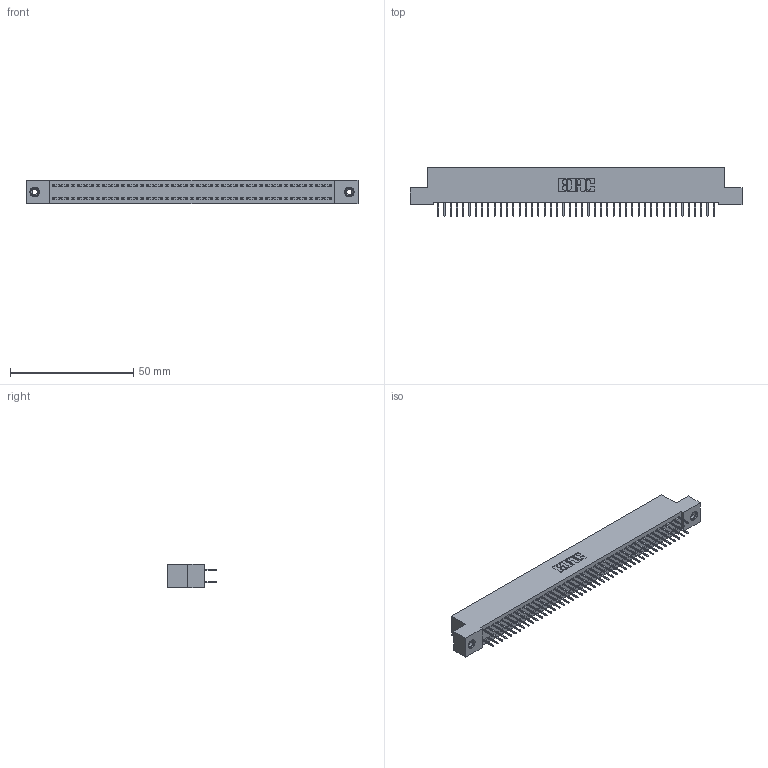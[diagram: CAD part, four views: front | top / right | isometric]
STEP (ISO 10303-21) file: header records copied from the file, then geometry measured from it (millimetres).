
FILE_DESCRIPTION (( 'STEP AP203' ), '1' );
FILE_NAME ('342-090-524-208.STEP', '2019-10-04T14:13:05', ( '' ), ( '' ), 'SwSTEP 2.0', 'SolidWorks 2016', '' );
FILE_SCHEMA (( 'CONFIG_CONTROL_DESIGN' ));
Length unit declared in the file: inch
Products named in the file (4): 345-292-001_345-293-124; 345-250-001_345-250-003-102; 342-090-524-208; 342 Part_TI
Assembly tree (93 placements, depth 2):
  342-090-524-208
    342 Part_TI
    345-292-001_345-293-124  x90
    345-250-001_345-250-003-102  x2
Bounding box: 134.62 x 19.69 x 9.4 mm (x, y, z)
Volume: 11967.9 mm3; surface area: 19210.7 mm2
Topology: 93 solids, 93 shells, 5210 faces, 14745 edges, 9462 vertices
Faces by surface type: plane 3878, cylinder 1316, cone 12, torus 4
Entity records: 29690 total; most frequent: CARTESIAN_POINT 4897, ORIENTED_EDGE 4826, DIRECTION 4211, EDGE_CURVE 2413, LINE 2269, VECTOR 2269, VERTEX_POINT 1600, AXIS2_PLACEMENT_3D 971
